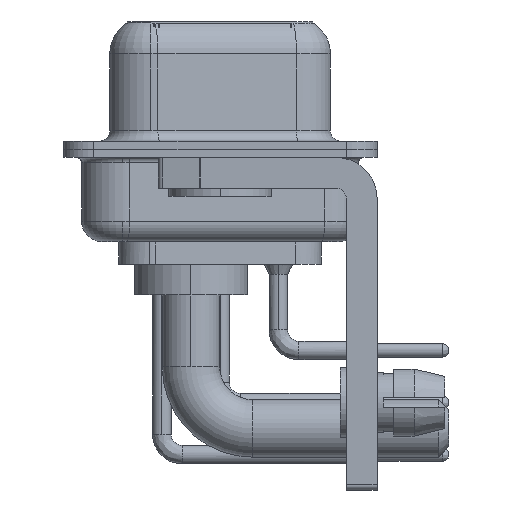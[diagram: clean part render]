
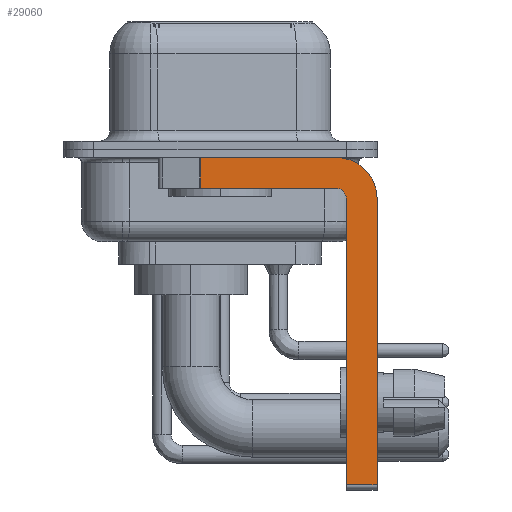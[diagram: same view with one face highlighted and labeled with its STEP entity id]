
A CAD part, left-side view. The second image highlights one B-rep face of the part: STEP entity #29060.
In plain terms, the highlighted planar face has unit normal (-1, 0, 0).
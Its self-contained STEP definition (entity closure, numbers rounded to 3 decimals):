
#137 = CARTESIAN_POINT ( 'NONE',  ( -2.9, -5.65, -2.4 ) ) ;
#1025 = LINE ( 'NONE', #17929, #8902 ) ;
#1119 = VERTEX_POINT ( 'NONE', #6666 ) ;
#1190 = CARTESIAN_POINT ( 'NONE',  ( -2.9, -7.65, -2.4 ) ) ;
#1504 = CIRCLE ( 'NONE', #25013, 0.5 ) ;
#2341 = AXIS2_PLACEMENT_3D ( 'NONE', #137, #11359, #22579 ) ;
#5134 = PLANE ( 'NONE',  #6491 ) ;
#5391 = EDGE_CURVE ( 'NONE', #20852, #20790, #1025, .T. ) ;
#5686 = VERTEX_POINT ( 'NONE', #8497 ) ;
#6491 = AXIS2_PLACEMENT_3D ( 'NONE', #35484, #22076, #10306 ) ;
#6666 = CARTESIAN_POINT ( 'NONE',  ( -2.9, 0.978, -1.9 ) ) ;
#7381 = CARTESIAN_POINT ( 'NONE',  ( -2.9, -5.65, -0.4 ) ) ;
#7834 = DIRECTION ( 'NONE',  ( 0., -1., 0. ) ) ;
#8497 = CARTESIAN_POINT ( 'NONE',  ( -2.9, -7.65, -16.35 ) ) ;
#8902 = VECTOR ( 'NONE', #29149, 1000. ) ;
#9177 = CARTESIAN_POINT ( 'NONE',  ( -2.9, -5.65, -1.9 ) ) ;
#10306 = DIRECTION ( 'NONE',  ( 0., 0., -1. ) ) ;
#10363 = VECTOR ( 'NONE', #31752, 1000. ) ;
#10378 = LINE ( 'NONE', #10563, #21554 ) ;
#10563 = CARTESIAN_POINT ( 'NONE',  ( -2.9, 3., -0.4 ) ) ;
#10614 = CARTESIAN_POINT ( 'NONE',  ( -2.9, -5.65, -16.35 ) ) ;
#11359 = DIRECTION ( 'NONE',  ( 1., 0., 0. ) ) ;
#11825 = VERTEX_POINT ( 'NONE', #9177 ) ;
#12192 = DIRECTION ( 'NONE',  ( -1., 0., 0. ) ) ;
#12673 = ORIENTED_EDGE ( 'NONE', *, *, #21156, .F. ) ;
#12913 = VERTEX_POINT ( 'NONE', #1190 ) ;
#13019 = CARTESIAN_POINT ( 'NONE',  ( -2.9, -6.15, -2.4 ) ) ;
#13069 = FACE_OUTER_BOUND ( 'NONE', #23099, .T. ) ;
#13728 = EDGE_CURVE ( 'NONE', #28074, #12913, #18202, .T. ) ;
#14221 = CARTESIAN_POINT ( 'NONE',  ( -2.9, -5.65, -1.9 ) ) ;
#14298 = LINE ( 'NONE', #23302, #31030 ) ;
#14480 = ORIENTED_EDGE ( 'NONE', *, *, #13728, .F. ) ;
#14788 = DIRECTION ( 'NONE',  ( 0., 0., 1. ) ) ;
#15262 = ORIENTED_EDGE ( 'NONE', *, *, #5391, .F. ) ;
#17017 = EDGE_CURVE ( 'NONE', #20790, #11825, #1504, .T. ) ;
#17929 = CARTESIAN_POINT ( 'NONE',  ( -2.9, -6.15, -16.6 ) ) ;
#18085 = EDGE_CURVE ( 'NONE', #23729, #1119, #25884, .T. ) ;
#18120 = EDGE_CURVE ( 'NONE', #23729, #28074, #10378, .T. ) ;
#18202 = CIRCLE ( 'NONE', #2341, 2. ) ;
#18953 = ORIENTED_EDGE ( 'NONE', *, *, #18085, .T. ) ;
#19702 = ORIENTED_EDGE ( 'NONE', *, *, #30196, .F. ) ;
#20721 = CARTESIAN_POINT ( 'NONE',  ( -2.9, 0.978, -1.9 ) ) ;
#20790 = VERTEX_POINT ( 'NONE', #13019 ) ;
#20852 = VERTEX_POINT ( 'NONE', #20943 ) ;
#20943 = CARTESIAN_POINT ( 'NONE',  ( -2.9, -6.15, -16.35 ) ) ;
#20982 = ORIENTED_EDGE ( 'NONE', *, *, #18120, .F. ) ;
#21058 = CARTESIAN_POINT ( 'NONE',  ( -2.9, 0.978, -0.4 ) ) ;
#21156 = EDGE_CURVE ( 'NONE', #12913, #5686, #14298, .T. ) ;
#21554 = VECTOR ( 'NONE', #29517, 1000. ) ;
#22055 = ORIENTED_EDGE ( 'NONE', *, *, #17017, .F. ) ;
#22076 = DIRECTION ( 'NONE',  ( 1., 0., 0. ) ) ;
#22579 = DIRECTION ( 'NONE',  ( 0., 0., -1. ) ) ;
#23099 = EDGE_LOOP ( 'NONE', ( #20982, #18953, #19702, #22055, #15262, #24892, #12673, #14480 ) ) ;
#23302 = CARTESIAN_POINT ( 'NONE',  ( -2.9, -7.65, -2.4 ) ) ;
#23418 = VECTOR ( 'NONE', #7834, 1000. ) ;
#23729 = VERTEX_POINT ( 'NONE', #21058 ) ;
#24892 = ORIENTED_EDGE ( 'NONE', *, *, #27096, .T. ) ;
#25013 = AXIS2_PLACEMENT_3D ( 'NONE', #33895, #12192, #14788 ) ;
#25429 = DIRECTION ( 'NONE',  ( 0., 1., 0. ) ) ;
#25884 = LINE ( 'NONE', #20721, #10363 ) ;
#27096 = EDGE_CURVE ( 'NONE', #20852, #5686, #35797, .T. ) ;
#28074 = VERTEX_POINT ( 'NONE', #7381 ) ;
#28451 = DIRECTION ( 'NONE',  ( 0., 0., -1. ) ) ;
#29060 = ADVANCED_FACE ( 'NONE', ( #13069 ), #5134, .F. ) ;
#29149 = DIRECTION ( 'NONE',  ( 0., 0., 1. ) ) ;
#29517 = DIRECTION ( 'NONE',  ( 0., -1., 0. ) ) ;
#30196 = EDGE_CURVE ( 'NONE', #11825, #1119, #30934, .T. ) ;
#30934 = LINE ( 'NONE', #14221, #34091 ) ;
#31030 = VECTOR ( 'NONE', #28451, 1000. ) ;
#31752 = DIRECTION ( 'NONE',  ( 0., 0., -1. ) ) ;
#33895 = CARTESIAN_POINT ( 'NONE',  ( -2.9, -5.65, -2.4 ) ) ;
#34091 = VECTOR ( 'NONE', #25429, 1000. ) ;
#35484 = CARTESIAN_POINT ( 'NONE',  ( -2.9, -5.65, -2.4 ) ) ;
#35797 = LINE ( 'NONE', #10614, #23418 ) ;
